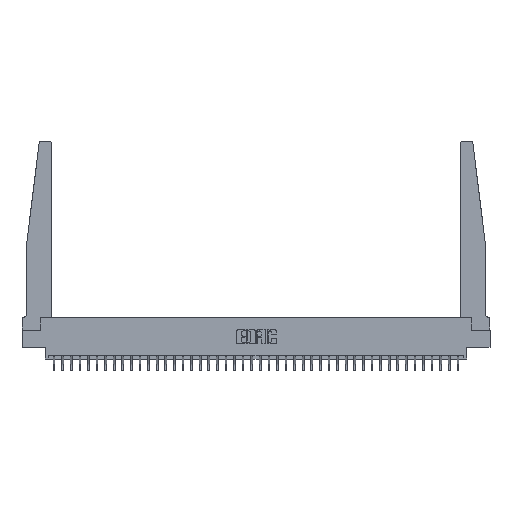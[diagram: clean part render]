
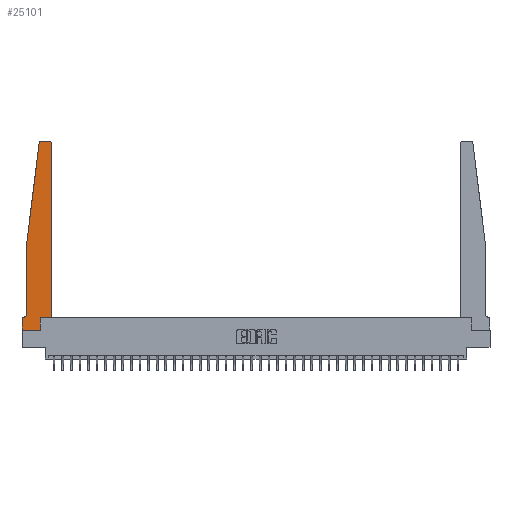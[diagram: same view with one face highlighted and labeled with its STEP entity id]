
A CAD part, top view. The second image highlights one B-rep face of the part: STEP entity #25101.
In plain terms, the highlighted planar face has unit normal (0, 0, 1).
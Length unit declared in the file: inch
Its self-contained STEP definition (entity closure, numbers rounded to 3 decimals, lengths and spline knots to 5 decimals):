
#83 = VECTOR ( 'NONE', #4479, 39.37008 ) ;
#226 = CARTESIAN_POINT ( 'NONE',  ( 0.2605, 0., 0.37 ) ) ;
#451 = DIRECTION ( 'NONE',  ( 0., 0., -1. ) ) ;
#1196 = ORIENTED_EDGE ( 'NONE', *, *, #4296, .T. ) ;
#1583 = DIRECTION ( 'NONE',  ( 1., 0., 0. ) ) ;
#1742 = CARTESIAN_POINT ( 'NONE',  ( 0., 0., 0.37 ) ) ;
#2337 = LINE ( 'NONE', #24663, #8798 ) ;
#2486 = ORIENTED_EDGE ( 'NONE', *, *, #7784, .T. ) ;
#3168 = VECTOR ( 'NONE', #13090, 39.37008 ) ;
#3195 = CARTESIAN_POINT ( 'NONE',  ( 0.015, 0.2375, 0.37 ) ) ;
#4240 = CARTESIAN_POINT ( 'NONE',  ( 0.065, 0.1875, 0.37 ) ) ;
#4296 = EDGE_CURVE ( 'NONE', #35379, #16115, #12367, .T. ) ;
#4338 = EDGE_CURVE ( 'NONE', #33018, #18793, #24603, .T. ) ;
#4479 = DIRECTION ( 'NONE',  ( 1., 0., 0. ) ) ;
#4704 = ORIENTED_EDGE ( 'NONE', *, *, #15817, .T. ) ;
#4892 = VERTEX_POINT ( 'NONE', #8449 ) ;
#5249 = FACE_OUTER_BOUND ( 'NONE', #15444, .T. ) ;
#5805 = EDGE_CURVE ( 'NONE', #28104, #18961, #9853, .T. ) ;
#6499 = EDGE_CURVE ( 'NONE', #12267, #28104, #2337, .T. ) ;
#6753 = CARTESIAN_POINT ( 'NONE',  ( 0.425, 0.18, 0.37 ) ) ;
#7784 = EDGE_CURVE ( 'NONE', #18961, #33018, #29666, .T. ) ;
#8046 = AXIS2_PLACEMENT_3D ( 'NONE', #24427, #26634, #18396 ) ;
#8444 = VECTOR ( 'NONE', #18516, 39.37008 ) ;
#8449 = CARTESIAN_POINT ( 'NONE',  ( 0.2605, 0.18, 0.37 ) ) ;
#8658 = EDGE_CURVE ( 'NONE', #18793, #17224, #12882, .T. ) ;
#8798 = VECTOR ( 'NONE', #17959, 39.37008 ) ;
#9062 = AXIS2_PLACEMENT_3D ( 'NONE', #26651, #35019, #1583 ) ;
#9418 = DIRECTION ( 'NONE',  ( 0., 0., 1. ) ) ;
#9468 = LINE ( 'NONE', #17508, #34865 ) ;
#9469 = AXIS2_PLACEMENT_3D ( 'NONE', #11818, #9418, #25549 ) ;
#9668 = ORIENTED_EDGE ( 'NONE', *, *, #6499, .T. ) ;
#9853 = CIRCLE ( 'NONE', #16277, 0.05 ) ;
#9979 = ORIENTED_EDGE ( 'NONE', *, *, #8658, .T. ) ;
#10766 = CARTESIAN_POINT ( 'NONE',  ( 0.425, 2.72, 0.37 ) ) ;
#11818 = CARTESIAN_POINT ( 'NONE',  ( 0., 0.1875, 0.37 ) ) ;
#11870 = ORIENTED_EDGE ( 'NONE', *, *, #4338, .T. ) ;
#12267 = VERTEX_POINT ( 'NONE', #23641 ) ;
#12337 = EDGE_CURVE ( 'NONE', #17224, #4892, #35303, .T. ) ;
#12367 = LINE ( 'NONE', #32289, #21290 ) ;
#12828 = CARTESIAN_POINT ( 'NONE',  ( 0., 0., 0.37 ) ) ;
#12882 = LINE ( 'NONE', #13067, #83 ) ;
#13067 = CARTESIAN_POINT ( 'NONE',  ( 0., 0., 0.37 ) ) ;
#13090 = DIRECTION ( 'NONE',  ( 0., -1., 0. ) ) ;
#13376 = ORIENTED_EDGE ( 'NONE', *, *, #12337, .T. ) ;
#14107 = DIRECTION ( 'NONE',  ( 1., 0., 0. ) ) ;
#14386 = PLANE ( 'NONE',  #9469 ) ;
#14967 = DIRECTION ( 'NONE',  ( -1., 0., 0. ) ) ;
#15145 = EDGE_CURVE ( 'NONE', #16115, #18629, #28945, .T. ) ;
#15444 = EDGE_LOOP ( 'NONE', ( #17288, #21052, #4704, #9668, #33914, #2486, #11870, #9979, #13376, #33593, #1196, #35246 ) ) ;
#15748 = DIRECTION ( 'NONE',  ( -1., 0., 0. ) ) ;
#15817 = EDGE_CURVE ( 'NONE', #32037, #12267, #20457, .T. ) ;
#16115 = VERTEX_POINT ( 'NONE', #10766 ) ;
#16277 = AXIS2_PLACEMENT_3D ( 'NONE', #3195, #451, #30982 ) ;
#16676 = CARTESIAN_POINT ( 'NONE',  ( 0.425, 0.18, 0.37 ) ) ;
#17224 = VERTEX_POINT ( 'NONE', #226 ) ;
#17288 = ORIENTED_EDGE ( 'NONE', *, *, #32929, .T. ) ;
#17508 = CARTESIAN_POINT ( 'NONE',  ( 0.25, 2.75, 0.37 ) ) ;
#17959 = DIRECTION ( 'NONE',  ( 0., -1., 0. ) ) ;
#18396 = DIRECTION ( 'NONE',  ( 1., 0., 0. ) ) ;
#18516 = DIRECTION ( 'NONE',  ( 0., 1., 0. ) ) ;
#18629 = VERTEX_POINT ( 'NONE', #22891 ) ;
#18793 = VERTEX_POINT ( 'NONE', #12828 ) ;
#18961 = VERTEX_POINT ( 'NONE', #30009 ) ;
#19375 = VERTEX_POINT ( 'NONE', #35963 ) ;
#20457 = LINE ( 'NONE', #22679, #32473 ) ;
#21052 = ORIENTED_EDGE ( 'NONE', *, *, #33520, .T. ) ;
#21290 = VECTOR ( 'NONE', #21320, 39.37008 ) ;
#21320 = DIRECTION ( 'NONE',  ( 0., 1., 0. ) ) ;
#22679 = CARTESIAN_POINT ( 'NONE',  ( 0.065, 1.25, 0.37 ) ) ;
#22891 = CARTESIAN_POINT ( 'NONE',  ( 0.395, 2.75, 0.37 ) ) ;
#22957 = CARTESIAN_POINT ( 'NONE',  ( 0.24675, 2.72367, 0.37 ) ) ;
#23641 = CARTESIAN_POINT ( 'NONE',  ( 0.065, 1.25, 0.37 ) ) ;
#23816 = CIRCLE ( 'NONE', #8046, 0.03 ) ;
#24427 = CARTESIAN_POINT ( 'NONE',  ( 0.27653, 2.72, 0.37 ) ) ;
#24603 = LINE ( 'NONE', #1742, #3168 ) ;
#24663 = CARTESIAN_POINT ( 'NONE',  ( 0.065, 1.25, 0.37 ) ) ;
#25101 = ADVANCED_FACE ( 'NONE', ( #5249 ), #14386, .T. ) ;
#25414 = VECTOR ( 'NONE', #14107, 39.37008 ) ;
#25549 = DIRECTION ( 'NONE',  ( 1., 0., 0. ) ) ;
#26634 = DIRECTION ( 'NONE',  ( 0., 0., 1. ) ) ;
#26651 = CARTESIAN_POINT ( 'NONE',  ( 0.395, 2.72, 0.37 ) ) ;
#26936 = VECTOR ( 'NONE', #15748, 39.37008 ) ;
#27465 = LINE ( 'NONE', #16676, #25414 ) ;
#28104 = VERTEX_POINT ( 'NONE', #30838 ) ;
#28371 = EDGE_CURVE ( 'NONE', #4892, #35379, #27465, .T. ) ;
#28693 = DIRECTION ( 'NONE',  ( -0.122, -0.992, 0. ) ) ;
#28945 = CIRCLE ( 'NONE', #9062, 0.03 ) ;
#29666 = LINE ( 'NONE', #4240, #26936 ) ;
#30009 = CARTESIAN_POINT ( 'NONE',  ( 0.015, 0.1875, 0.37 ) ) ;
#30838 = CARTESIAN_POINT ( 'NONE',  ( 0.065, 0.2375, 0.37 ) ) ;
#30982 = DIRECTION ( 'NONE',  ( -1., 0., 0. ) ) ;
#32037 = VERTEX_POINT ( 'NONE', #22957 ) ;
#32215 = CARTESIAN_POINT ( 'NONE',  ( 0.2605, 0.18, 0.37 ) ) ;
#32289 = CARTESIAN_POINT ( 'NONE',  ( 0.425, 0.18, 0.37 ) ) ;
#32473 = VECTOR ( 'NONE', #28693, 39.37008 ) ;
#32929 = EDGE_CURVE ( 'NONE', #18629, #19375, #9468, .T. ) ;
#33018 = VERTEX_POINT ( 'NONE', #34699 ) ;
#33520 = EDGE_CURVE ( 'NONE', #19375, #32037, #23816, .T. ) ;
#33593 = ORIENTED_EDGE ( 'NONE', *, *, #28371, .T. ) ;
#33914 = ORIENTED_EDGE ( 'NONE', *, *, #5805, .T. ) ;
#34699 = CARTESIAN_POINT ( 'NONE',  ( 0., 0.1875, 0.37 ) ) ;
#34865 = VECTOR ( 'NONE', #14967, 39.37008 ) ;
#35019 = DIRECTION ( 'NONE',  ( 0., 0., 1. ) ) ;
#35246 = ORIENTED_EDGE ( 'NONE', *, *, #15145, .T. ) ;
#35303 = LINE ( 'NONE', #32215, #8444 ) ;
#35379 = VERTEX_POINT ( 'NONE', #6753 ) ;
#35963 = CARTESIAN_POINT ( 'NONE',  ( 0.27653, 2.75, 0.37 ) ) ;
